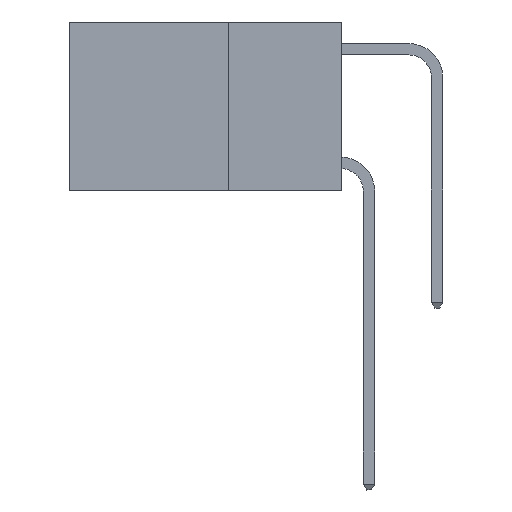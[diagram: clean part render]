
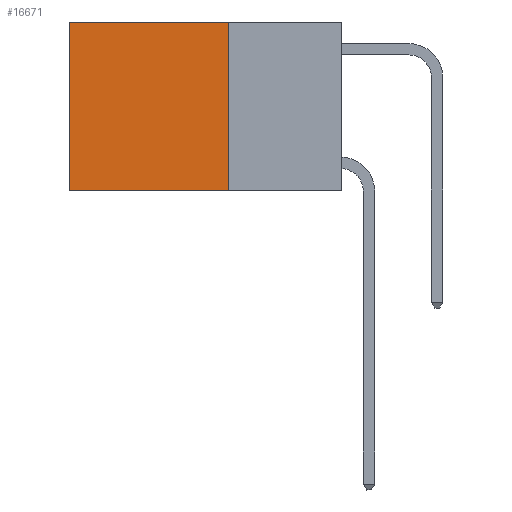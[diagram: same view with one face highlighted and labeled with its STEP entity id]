
A CAD part, left-side view. The second image highlights one B-rep face of the part: STEP entity #16671.
In plain terms, the highlighted planar face has unit normal (-1, 0, 0).
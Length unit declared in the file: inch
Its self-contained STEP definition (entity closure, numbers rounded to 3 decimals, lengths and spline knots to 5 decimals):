
#1673 = DIRECTION ( 'NONE',  ( 0., 1., 0. ) ) ;
#2556 = ORIENTED_EDGE ( 'NONE', *, *, #18445, .F. ) ;
#3009 = CARTESIAN_POINT ( 'NONE',  ( 0.2625, 0.25, -0.37 ) ) ;
#3287 = VECTOR ( 'NONE', #7940, 39.37008 ) ;
#3351 = CARTESIAN_POINT ( 'NONE',  ( 0.2625, 0.25, 0. ) ) ;
#4147 = LINE ( 'NONE', #5801, #19749 ) ;
#4167 = VERTEX_POINT ( 'NONE', #3009 ) ;
#4773 = FACE_OUTER_BOUND ( 'NONE', #20959, .T. ) ;
#4849 = CARTESIAN_POINT ( 'NONE',  ( 0.2625, 0.25, 0. ) ) ;
#5474 = DIRECTION ( 'NONE',  ( 0., 0., -1. ) ) ;
#5595 = VECTOR ( 'NONE', #1673, 39.37008 ) ;
#5801 = CARTESIAN_POINT ( 'NONE',  ( 0.2625, 0.6, 0. ) ) ;
#6304 = ORIENTED_EDGE ( 'NONE', *, *, #9492, .T. ) ;
#7940 = DIRECTION ( 'NONE',  ( 0., 1., 0. ) ) ;
#8038 = LINE ( 'NONE', #16363, #5595 ) ;
#8069 = CARTESIAN_POINT ( 'NONE',  ( 0.2625, 0.25, 0. ) ) ;
#9084 = AXIS2_PLACEMENT_3D ( 'NONE', #8069, #11437, #21300 ) ;
#9214 = ORIENTED_EDGE ( 'NONE', *, *, #18461, .F. ) ;
#9490 = CARTESIAN_POINT ( 'NONE',  ( 0.2625, 0.6, -0.37 ) ) ;
#9492 = EDGE_CURVE ( 'NONE', #19524, #16405, #12969, .T. ) ;
#9682 = DIRECTION ( 'NONE',  ( 0., 0., -1. ) ) ;
#9716 = PLANE ( 'NONE',  #9084 ) ;
#10263 = CARTESIAN_POINT ( 'NONE',  ( 0.2625, 0.6, 0. ) ) ;
#10484 = VECTOR ( 'NONE', #9682, 39.37008 ) ;
#10861 = EDGE_CURVE ( 'NONE', #16405, #15341, #4147, .T. ) ;
#11437 = DIRECTION ( 'NONE',  ( 1., 0., 0. ) ) ;
#12969 = LINE ( 'NONE', #14405, #3287 ) ;
#14405 = CARTESIAN_POINT ( 'NONE',  ( 0.2625, 0.25, 0. ) ) ;
#15341 = VERTEX_POINT ( 'NONE', #9490 ) ;
#16363 = CARTESIAN_POINT ( 'NONE',  ( 0.2625, 0.25, -0.37 ) ) ;
#16405 = VERTEX_POINT ( 'NONE', #10263 ) ;
#16471 = LINE ( 'NONE', #4849, #10484 ) ;
#16671 = ADVANCED_FACE ( 'NONE', ( #4773 ), #9716, .F. ) ;
#18445 = EDGE_CURVE ( 'NONE', #19524, #4167, #16471, .T. ) ;
#18461 = EDGE_CURVE ( 'NONE', #4167, #15341, #8038, .T. ) ;
#19524 = VERTEX_POINT ( 'NONE', #3351 ) ;
#19749 = VECTOR ( 'NONE', #5474, 39.37008 ) ;
#20658 = ORIENTED_EDGE ( 'NONE', *, *, #10861, .T. ) ;
#20959 = EDGE_LOOP ( 'NONE', ( #20658, #9214, #2556, #6304 ) ) ;
#21300 = DIRECTION ( 'NONE',  ( 0., 0., -1. ) ) ;
